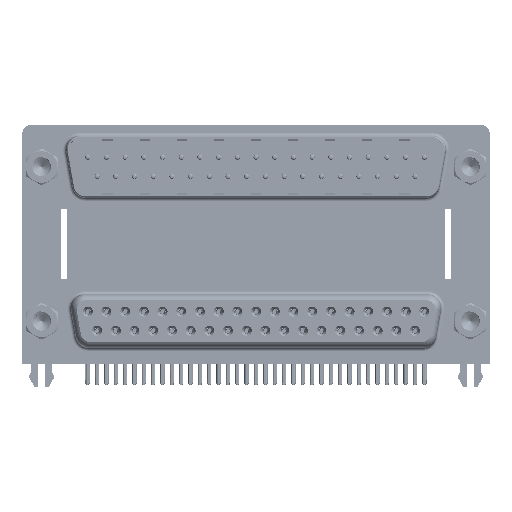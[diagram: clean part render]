
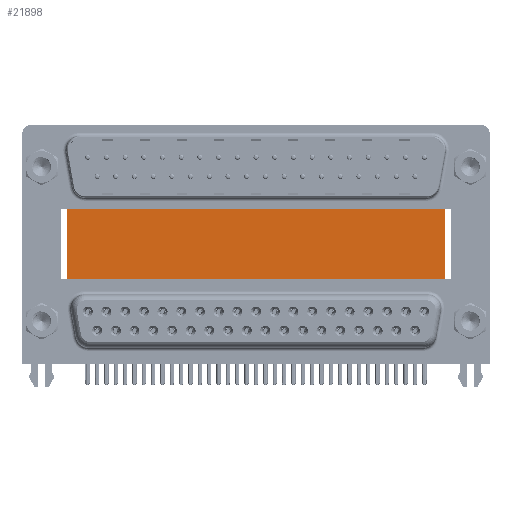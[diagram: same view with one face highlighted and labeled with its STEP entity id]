
A CAD part, top view. The second image highlights one B-rep face of the part: STEP entity #21898.
In plain terms, the highlighted planar face has unit normal (0, 0, 1).
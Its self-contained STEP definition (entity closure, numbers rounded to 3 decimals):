
#2652 = LINE ( 'NONE', #42885, #71948 ) ;
#4399 = VECTOR ( 'NONE', #54589, 1000. ) ;
#5971 = VECTOR ( 'NONE', #55770, 1000. ) ;
#9128 = LINE ( 'NONE', #61008, #25763 ) ;
#9336 = PLANE ( 'NONE',  #73496 ) ;
#9845 = LINE ( 'NONE', #31638, #4399 ) ;
#10387 = VERTEX_POINT ( 'NONE', #14386 ) ;
#10774 = EDGE_LOOP ( 'NONE', ( #60393, #20401, #13333, #53224 ) ) ;
#12052 = LINE ( 'NONE', #51887, #5971 ) ;
#12209 = VERTEX_POINT ( 'NONE', #32662 ) ;
#13333 = ORIENTED_EDGE ( 'NONE', *, *, #61579, .F. ) ;
#13826 = VERTEX_POINT ( 'NONE', #17997 ) ;
#14386 = CARTESIAN_POINT ( 'NONE',  ( 59.71, -3.735, -12. ) ) ;
#15517 = DIRECTION ( 'NONE',  ( 0., -1., 0. ) ) ;
#17997 = CARTESIAN_POINT ( 'NONE',  ( 59.71, 16.585, -12. ) ) ;
#18252 = EDGE_CURVE ( 'NONE', #12209, #65341, #2652, .T. ) ;
#20335 = DIRECTION ( 'NONE',  ( 0., -1., 0. ) ) ;
#20401 = ORIENTED_EDGE ( 'NONE', *, *, #41794, .F. ) ;
#21335 = DIRECTION ( 'NONE',  ( 0., 0., -1. ) ) ;
#21898 = ADVANCED_FACE ( 'NONE', ( #72529 ), #9336, .F. ) ;
#25763 = VECTOR ( 'NONE', #15517, 1000. ) ;
#31638 = CARTESIAN_POINT ( 'NONE',  ( 3.79, -3.735, -12. ) ) ;
#32041 = CARTESIAN_POINT ( 'NONE',  ( 3.79, -3.735, -12. ) ) ;
#32662 = CARTESIAN_POINT ( 'NONE',  ( 3.79, 16.585, -12. ) ) ;
#37905 = DIRECTION ( 'NONE',  ( -1., 0., 0. ) ) ;
#41794 = EDGE_CURVE ( 'NONE', #13826, #10387, #9128, .T. ) ;
#42799 = CARTESIAN_POINT ( 'NONE',  ( 3.79, 16.585, -12. ) ) ;
#42885 = CARTESIAN_POINT ( 'NONE',  ( 3.79, 16.585, -12. ) ) ;
#51887 = CARTESIAN_POINT ( 'NONE',  ( 3.79, 16.585, -12. ) ) ;
#53224 = ORIENTED_EDGE ( 'NONE', *, *, #18252, .T. ) ;
#54589 = DIRECTION ( 'NONE',  ( 1., 0., 0. ) ) ;
#55770 = DIRECTION ( 'NONE',  ( 1., 0., 0. ) ) ;
#55922 = EDGE_CURVE ( 'NONE', #65341, #10387, #9845, .T. ) ;
#60393 = ORIENTED_EDGE ( 'NONE', *, *, #55922, .T. ) ;
#61008 = CARTESIAN_POINT ( 'NONE',  ( 59.71, 16.585, -12. ) ) ;
#61579 = EDGE_CURVE ( 'NONE', #12209, #13826, #12052, .T. ) ;
#65341 = VERTEX_POINT ( 'NONE', #32041 ) ;
#71948 = VECTOR ( 'NONE', #20335, 1000. ) ;
#72529 = FACE_OUTER_BOUND ( 'NONE', #10774, .T. ) ;
#73496 = AXIS2_PLACEMENT_3D ( 'NONE', #42799, #21335, #37905 ) ;
